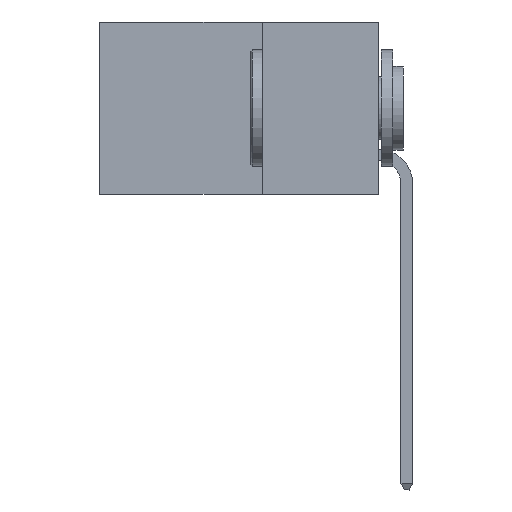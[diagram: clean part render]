
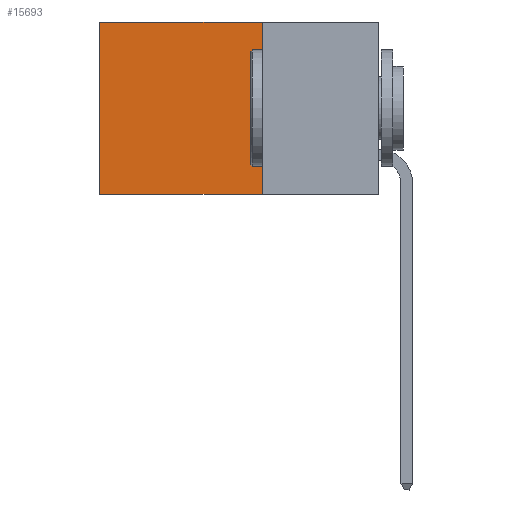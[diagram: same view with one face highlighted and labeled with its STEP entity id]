
A CAD part, left-side view. The second image highlights one B-rep face of the part: STEP entity #15693.
In plain terms, the highlighted planar face has unit normal (-1, 0, 0).
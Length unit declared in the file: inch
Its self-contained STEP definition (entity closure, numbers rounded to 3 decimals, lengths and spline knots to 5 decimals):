
#378 = LINE ( 'NONE', #4033, #9567 ) ;
#1061 = VECTOR ( 'NONE', #16762, 39.37008 ) ;
#1536 = FACE_OUTER_BOUND ( 'NONE', #13161, .T. ) ;
#2440 = ORIENTED_EDGE ( 'NONE', *, *, #8360, .F. ) ;
#2746 = VECTOR ( 'NONE', #17314, 39.37008 ) ;
#2762 = EDGE_CURVE ( 'NONE', #17181, #11313, #9426, .T. ) ;
#3785 = PLANE ( 'NONE',  #4738 ) ;
#3946 = CARTESIAN_POINT ( 'NONE',  ( 0.298, 0.25, 0. ) ) ;
#4033 = CARTESIAN_POINT ( 'NONE',  ( 0.298, 0.6, 0. ) ) ;
#4738 = AXIS2_PLACEMENT_3D ( 'NONE', #5254, #6715, #17021 ) ;
#5254 = CARTESIAN_POINT ( 'NONE',  ( 0.298, 0.25, 0. ) ) ;
#5372 = EDGE_CURVE ( 'NONE', #10611, #13658, #378, .T. ) ;
#6436 = ORIENTED_EDGE ( 'NONE', *, *, #5372, .T. ) ;
#6715 = DIRECTION ( 'NONE',  ( 1., 0., 0. ) ) ;
#6785 = CARTESIAN_POINT ( 'NONE',  ( 0.298, 0.6, 0. ) ) ;
#7093 = CARTESIAN_POINT ( 'NONE',  ( 0.298, 0.25, -0.37 ) ) ;
#8360 = EDGE_CURVE ( 'NONE', #11313, #13658, #13108, .T. ) ;
#8503 = DIRECTION ( 'NONE',  ( 0., 0., -1. ) ) ;
#9426 = LINE ( 'NONE', #3946, #2746 ) ;
#9550 = CARTESIAN_POINT ( 'NONE',  ( 0.298, 0.6, -0.37 ) ) ;
#9567 = VECTOR ( 'NONE', #8503, 39.37008 ) ;
#10611 = VERTEX_POINT ( 'NONE', #6785 ) ;
#10880 = CARTESIAN_POINT ( 'NONE',  ( 0.298, 0.25, 0. ) ) ;
#10896 = EDGE_CURVE ( 'NONE', #17181, #10611, #17641, .T. ) ;
#11174 = ORIENTED_EDGE ( 'NONE', *, *, #2762, .F. ) ;
#11313 = VERTEX_POINT ( 'NONE', #17910 ) ;
#13108 = LINE ( 'NONE', #7093, #15880 ) ;
#13161 = EDGE_LOOP ( 'NONE', ( #6436, #2440, #11174, #14593 ) ) ;
#13658 = VERTEX_POINT ( 'NONE', #9550 ) ;
#14525 = DIRECTION ( 'NONE',  ( 0., 1., 0. ) ) ;
#14593 = ORIENTED_EDGE ( 'NONE', *, *, #10896, .T. ) ;
#15693 = ADVANCED_FACE ( 'NONE', ( #1536 ), #3785, .F. ) ;
#15880 = VECTOR ( 'NONE', #14525, 39.37008 ) ;
#16762 = DIRECTION ( 'NONE',  ( 0., 1., 0. ) ) ;
#17021 = DIRECTION ( 'NONE',  ( 0., 0., -1. ) ) ;
#17181 = VERTEX_POINT ( 'NONE', #17382 ) ;
#17314 = DIRECTION ( 'NONE',  ( 0., 0., -1. ) ) ;
#17382 = CARTESIAN_POINT ( 'NONE',  ( 0.298, 0.25, 0. ) ) ;
#17641 = LINE ( 'NONE', #10880, #1061 ) ;
#17910 = CARTESIAN_POINT ( 'NONE',  ( 0.298, 0.25, -0.37 ) ) ;
